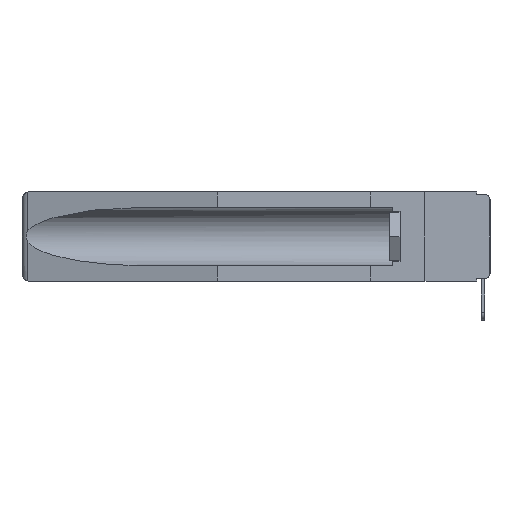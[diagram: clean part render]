
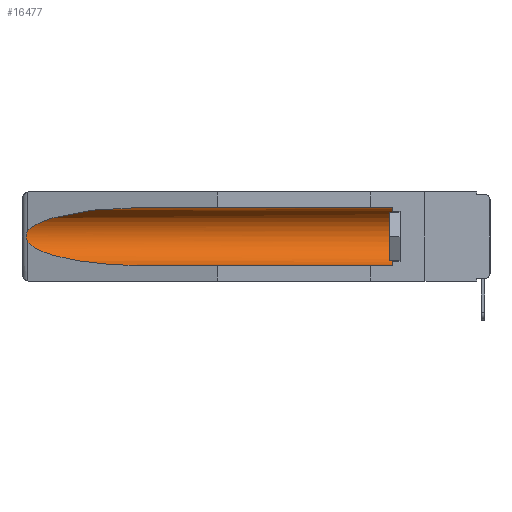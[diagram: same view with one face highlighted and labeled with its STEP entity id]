
A CAD part, left-side view. The second image highlights one B-rep face of the part: STEP entity #16477.
In plain terms, the highlighted cylindrical face has radius 2.857 mm (diameter 5.715 mm), a partial arc.
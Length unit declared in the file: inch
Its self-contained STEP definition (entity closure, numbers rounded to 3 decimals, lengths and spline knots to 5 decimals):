
#346 = VERTEX_POINT ( 'NONE', #13149 ) ;
#638 = CIRCLE ( 'NONE', #7342, 0.1125 ) ;
#879 = CARTESIAN_POINT ( 'NONE',  ( 0.26537, 1.52718, -0.14972 ) ) ;
#1194 =( BOUNDED_CURVE ( )  B_SPLINE_CURVE ( 3, ( #19089, #12933, #4820, #23632 ),
 .UNSPECIFIED., .F., .F. ) 
 B_SPLINE_CURVE_WITH_KNOTS ( ( 4, 4 ),
 ( 4.71239, 6.08839 ),
 .UNSPECIFIED. ) 
 CURVE ( )  GEOMETRIC_REPRESENTATION_ITEM ( )  RATIONAL_B_SPLINE_CURVE ( ( 1., 0.848, 0.848, 1. ) ) 
 REPRESENTATION_ITEM ( '' )  );
#1311 = DIRECTION ( 'NONE',  ( 0., 1., 0. ) ) ;
#1686 = EDGE_CURVE ( 'NONE', #6581, #15631, #1194, .T. ) ;
#2018 =( BOUNDED_CURVE ( )  B_SPLINE_CURVE ( 3, ( #15933, #24354, #9755, #11934 ),
 .UNSPECIFIED., .F., .F. ) 
 B_SPLINE_CURVE_WITH_KNOTS ( ( 4, 4 ),
 ( 0.1948, 1.5708 ),
 .UNSPECIFIED. ) 
 CURVE ( )  GEOMETRIC_REPRESENTATION_ITEM ( )  RATIONAL_B_SPLINE_CURVE ( ( 1., 0.848, 0.848, 1. ) ) 
 REPRESENTATION_ITEM ( '' )  );
#2284 = CARTESIAN_POINT ( 'NONE',  ( 0.26655, 1.53094, -0.18657 ) ) ;
#2831 = AXIS2_PLACEMENT_3D ( 'NONE', #7527, #1311, #11967 ) ;
#3316 = ORIENTED_EDGE ( 'NONE', *, *, #19983, .T. ) ;
#4203 = CARTESIAN_POINT ( 'NONE',  ( 0.26597, 1.52961, -0.15275 ) ) ;
#4820 = CARTESIAN_POINT ( 'NONE',  ( 0.25451, 1.48313, -0.09465 ) ) ;
#5383 = CARTESIAN_POINT ( 'NONE',  ( 0.155, 0.126, -0.1715 ) ) ;
#6581 = VERTEX_POINT ( 'NONE', #21873 ) ;
#6587 = EDGE_CURVE ( 'NONE', #20137, #22620, #20345, .T. ) ;
#7220 = CARTESIAN_POINT ( 'NONE',  ( 0.155, 1.07973, -0.284 ) ) ;
#7342 = AXIS2_PLACEMENT_3D ( 'NONE', #5383, #19907, #13580 ) ;
#7345 = CYLINDRICAL_SURFACE ( 'NONE', #2831, 0.1125 ) ;
#7527 = CARTESIAN_POINT ( 'NONE',  ( 0.155, -0.30754, -0.1715 ) ) ;
#8213 = CARTESIAN_POINT ( 'NONE',  ( 0.155, 0.126, -0.284 ) ) ;
#8420 = CARTESIAN_POINT ( 'NONE',  ( 0.2673, 1.53269, -0.17917 ) ) ;
#9755 = CARTESIAN_POINT ( 'NONE',  ( 0.21114, 1.30732, -0.284 ) ) ;
#10766 = CARTESIAN_POINT ( 'NONE',  ( 0.2675, 1.53308, -0.16763 ) ) ;
#10844 = CARTESIAN_POINT ( 'NONE',  ( 0.26597, 1.5296, -0.19026 ) ) ;
#10900 = FACE_OUTER_BOUND ( 'NONE', #17128, .T. ) ;
#11708 = DIRECTION ( 'NONE',  ( 0., 1., 0. ) ) ;
#11934 = CARTESIAN_POINT ( 'NONE',  ( 0.155, 1.07973, -0.284 ) ) ;
#11967 = DIRECTION ( 'NONE',  ( 0., 0., 1. ) ) ;
#12075 = ORIENTED_EDGE ( 'NONE', *, *, #22537, .T. ) ;
#12339 = DIRECTION ( 'NONE',  ( 0., 1., 0. ) ) ;
#12933 = CARTESIAN_POINT ( 'NONE',  ( 0.21114, 1.30732, -0.059 ) ) ;
#13149 = CARTESIAN_POINT ( 'NONE',  ( 0.26537, 1.52718, -0.19328 ) ) ;
#13455 = CARTESIAN_POINT ( 'NONE',  ( 0.155, -0.30754, -0.284 ) ) ;
#13580 = DIRECTION ( 'NONE',  ( 0., 0., 1. ) ) ;
#14286 = ORIENTED_EDGE ( 'NONE', *, *, #22295, .T. ) ;
#14747 = EDGE_CURVE ( 'NONE', #23314, #6581, #25418, .T. ) ;
#14765 = CARTESIAN_POINT ( 'NONE',  ( 0.26537, 1.52718, -0.14972 ) ) ;
#14901 = CARTESIAN_POINT ( 'NONE',  ( 0.155, 0.126, -0.059 ) ) ;
#15012 = ORIENTED_EDGE ( 'NONE', *, *, #14747, .T. ) ;
#15478 = VECTOR ( 'NONE', #11708, 39.37008 ) ;
#15631 = VERTEX_POINT ( 'NONE', #879 ) ;
#15933 = CARTESIAN_POINT ( 'NONE',  ( 0.26537, 1.52718, -0.19328 ) ) ;
#16477 = ADVANCED_FACE ( 'NONE', ( #10900 ), #7345, .F. ) ;
#16691 = ORIENTED_EDGE ( 'NONE', *, *, #1686, .T. ) ;
#17128 = EDGE_LOOP ( 'NONE', ( #16691, #14286, #3316, #26319, #12075, #15012 ) ) ;
#18746 = CARTESIAN_POINT ( 'NONE',  ( 0.2675, 1.53308, -0.17534 ) ) ;
#19089 = CARTESIAN_POINT ( 'NONE',  ( 0.155, 1.07973, -0.059 ) ) ;
#19104 = CARTESIAN_POINT ( 'NONE',  ( 0.26654, 1.53092, -0.15636 ) ) ;
#19907 = DIRECTION ( 'NONE',  ( 0., -1., 0. ) ) ;
#19983 = EDGE_CURVE ( 'NONE', #346, #22620, #2018, .T. ) ;
#20137 = VERTEX_POINT ( 'NONE', #8213 ) ;
#20345 = LINE ( 'NONE', #13455, #15478 ) ;
#20578 = CARTESIAN_POINT ( 'NONE',  ( 0.155, -0.30754, -0.059 ) ) ;
#21015 = B_SPLINE_CURVE_WITH_KNOTS ( 'NONE', 3,
 ( #14765, #4203, #19104, #23028, #10766, #18746, #8420, #2284, #10844, #25360 ),
 .UNSPECIFIED., .F., .F.,
 ( 4, 2, 2, 2, 4 ),
 ( 0., 0.00029, 0.00058, 0.00087, 0.00117 ),
 .UNSPECIFIED. ) ;
#21508 = VECTOR ( 'NONE', #12339, 39.37008 ) ;
#21873 = CARTESIAN_POINT ( 'NONE',  ( 0.155, 1.07973, -0.059 ) ) ;
#22295 = EDGE_CURVE ( 'NONE', #15631, #346, #21015, .T. ) ;
#22537 = EDGE_CURVE ( 'NONE', #20137, #23314, #638, .T. ) ;
#22620 = VERTEX_POINT ( 'NONE', #7220 ) ;
#23028 = CARTESIAN_POINT ( 'NONE',  ( 0.2673, 1.5327, -0.16383 ) ) ;
#23314 = VERTEX_POINT ( 'NONE', #14901 ) ;
#23632 = CARTESIAN_POINT ( 'NONE',  ( 0.26537, 1.52718, -0.14972 ) ) ;
#24354 = CARTESIAN_POINT ( 'NONE',  ( 0.25451, 1.48313, -0.24835 ) ) ;
#25360 = CARTESIAN_POINT ( 'NONE',  ( 0.26537, 1.52718, -0.19328 ) ) ;
#25418 = LINE ( 'NONE', #20578, #21508 ) ;
#26319 = ORIENTED_EDGE ( 'NONE', *, *, #6587, .F. ) ;
